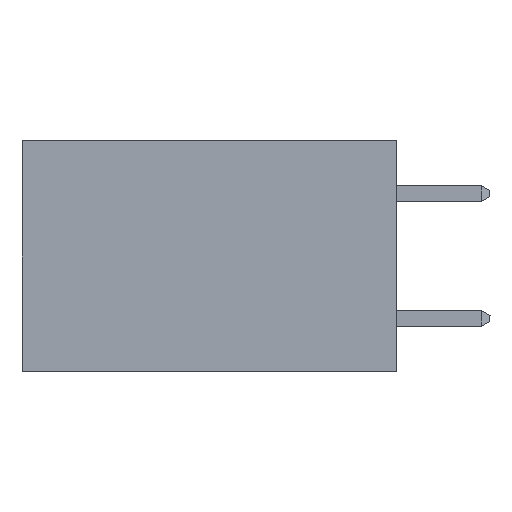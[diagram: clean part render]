
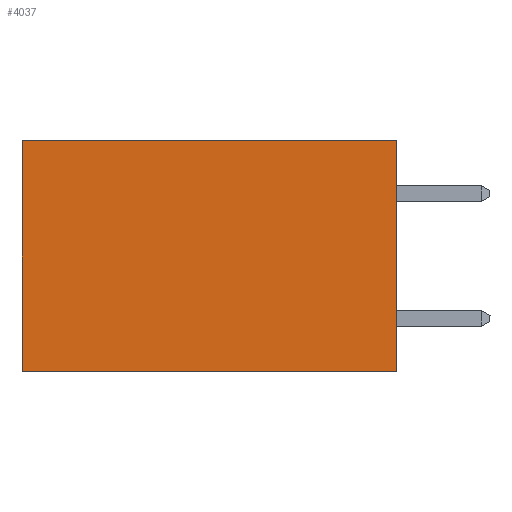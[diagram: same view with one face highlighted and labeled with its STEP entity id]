
A CAD part, left-side view. The second image highlights one B-rep face of the part: STEP entity #4037.
In plain terms, the highlighted planar face has unit normal (-1, 0, 0).
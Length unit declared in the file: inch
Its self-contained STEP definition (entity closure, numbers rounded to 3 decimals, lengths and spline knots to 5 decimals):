
#119 = ORIENTED_EDGE ( 'NONE', *, *, #8380, .T. ) ;
#488 = FACE_OUTER_BOUND ( 'NONE', #15539, .T. ) ;
#956 = LINE ( 'NONE', #6190, #4536 ) ;
#1032 = PLANE ( 'NONE',  #4990 ) ;
#1073 = CARTESIAN_POINT ( 'NONE',  ( 0.2615, 0., -0.37 ) ) ;
#2029 = VECTOR ( 'NONE', #16703, 39.37008 ) ;
#2087 = VECTOR ( 'NONE', #8805, 39.37008 ) ;
#4037 = ADVANCED_FACE ( 'NONE', ( #488 ), #1032, .F. ) ;
#4536 = VECTOR ( 'NONE', #12734, 39.37008 ) ;
#4789 = EDGE_CURVE ( 'NONE', #8672, #8471, #16318, .T. ) ;
#4990 = AXIS2_PLACEMENT_3D ( 'NONE', #16931, #16874, #16711 ) ;
#5689 = LINE ( 'NONE', #13284, #11411 ) ;
#5967 = EDGE_CURVE ( 'NONE', #8471, #10504, #5689, .T. ) ;
#5971 = CARTESIAN_POINT ( 'NONE',  ( 0.2615, 0.6, 0. ) ) ;
#6190 = CARTESIAN_POINT ( 'NONE',  ( 0.2615, 0., 0. ) ) ;
#6516 = CARTESIAN_POINT ( 'NONE',  ( 0.2615, 0.6, -0.37 ) ) ;
#6537 = EDGE_CURVE ( 'NONE', #10171, #10504, #9016, .T. ) ;
#8380 = EDGE_CURVE ( 'NONE', #8672, #10171, #956, .T. ) ;
#8471 = VERTEX_POINT ( 'NONE', #1073 ) ;
#8672 = VERTEX_POINT ( 'NONE', #12025 ) ;
#8805 = DIRECTION ( 'NONE',  ( 0., 0., -1. ) ) ;
#8960 = CARTESIAN_POINT ( 'NONE',  ( 0.2615, 0.6, -0.37 ) ) ;
#9016 = LINE ( 'NONE', #8960, #2087 ) ;
#9560 = ORIENTED_EDGE ( 'NONE', *, *, #5967, .F. ) ;
#10171 = VERTEX_POINT ( 'NONE', #5971 ) ;
#10504 = VERTEX_POINT ( 'NONE', #6516 ) ;
#11345 = ORIENTED_EDGE ( 'NONE', *, *, #6537, .T. ) ;
#11411 = VECTOR ( 'NONE', #13220, 39.37008 ) ;
#12025 = CARTESIAN_POINT ( 'NONE',  ( 0.2615, 0., 0. ) ) ;
#12174 = ORIENTED_EDGE ( 'NONE', *, *, #4789, .F. ) ;
#12734 = DIRECTION ( 'NONE',  ( 0., 1., 0. ) ) ;
#13220 = DIRECTION ( 'NONE',  ( 0., 1., 0. ) ) ;
#13284 = CARTESIAN_POINT ( 'NONE',  ( 0.2615, 0., -0.37 ) ) ;
#15539 = EDGE_LOOP ( 'NONE', ( #11345, #9560, #12174, #119 ) ) ;
#15731 = CARTESIAN_POINT ( 'NONE',  ( 0.2615, 0., -0.37 ) ) ;
#16318 = LINE ( 'NONE', #15731, #2029 ) ;
#16703 = DIRECTION ( 'NONE',  ( 0., 0., -1. ) ) ;
#16711 = DIRECTION ( 'NONE',  ( 0., 0., -1. ) ) ;
#16874 = DIRECTION ( 'NONE',  ( 1., 0., 0. ) ) ;
#16931 = CARTESIAN_POINT ( 'NONE',  ( 0.2615, 0., -0.37 ) ) ;
